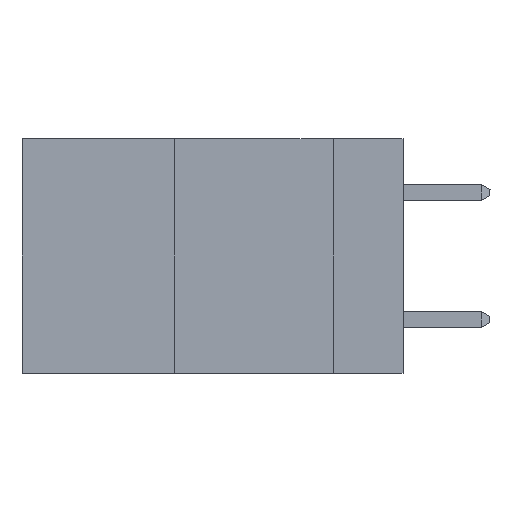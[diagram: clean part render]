
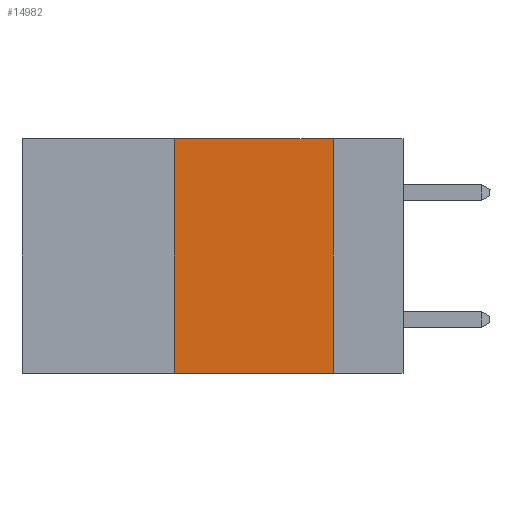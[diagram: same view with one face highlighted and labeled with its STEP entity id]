
A CAD part, left-side view. The second image highlights one B-rep face of the part: STEP entity #14982.
In plain terms, the highlighted planar face has unit normal (-1, 0, 0).
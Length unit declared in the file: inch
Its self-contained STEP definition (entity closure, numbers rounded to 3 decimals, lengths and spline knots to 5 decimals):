
#1082 = AXIS2_PLACEMENT_3D ( 'NONE', #10005, #19451, #3725 ) ;
#1822 = CARTESIAN_POINT ( 'NONE',  ( 0., 0.11, 0. ) ) ;
#2431 = DIRECTION ( 'NONE',  ( 0., -1., 0. ) ) ;
#2682 = EDGE_CURVE ( 'NONE', #5881, #14413, #19854, .T. ) ;
#3580 = CARTESIAN_POINT ( 'NONE',  ( 0., 0.11, -0.37 ) ) ;
#3661 = PLANE ( 'NONE',  #1082 ) ;
#3725 = DIRECTION ( 'NONE',  ( 0., 0., -1. ) ) ;
#3844 = LINE ( 'NONE', #13493, #9092 ) ;
#3905 = FACE_OUTER_BOUND ( 'NONE', #15413, .T. ) ;
#4146 = CARTESIAN_POINT ( 'NONE',  ( 0., 0.6, 0. ) ) ;
#5061 = VECTOR ( 'NONE', #5897, 39.37008 ) ;
#5077 = ORIENTED_EDGE ( 'NONE', *, *, #10117, .F. ) ;
#5511 = DIRECTION ( 'NONE',  ( 0., 0., -1. ) ) ;
#5881 = VERTEX_POINT ( 'NONE', #6553 ) ;
#5897 = DIRECTION ( 'NONE',  ( 0., -1., 0. ) ) ;
#6307 = CARTESIAN_POINT ( 'NONE',  ( 0., 0.36, 0. ) ) ;
#6553 = CARTESIAN_POINT ( 'NONE',  ( 0., 0.36, 0. ) ) ;
#8255 = EDGE_CURVE ( 'NONE', #11700, #13579, #10612, .T. ) ;
#8374 = DIRECTION ( 'NONE',  ( 0., 0., 1. ) ) ;
#9092 = VECTOR ( 'NONE', #5511, 39.37008 ) ;
#10005 = CARTESIAN_POINT ( 'NONE',  ( 0., 0.6, 0. ) ) ;
#10117 = EDGE_CURVE ( 'NONE', #14413, #13579, #3844, .T. ) ;
#10612 = LINE ( 'NONE', #15279, #5061 ) ;
#11083 = ORIENTED_EDGE ( 'NONE', *, *, #2682, .F. ) ;
#11700 = VERTEX_POINT ( 'NONE', #14777 ) ;
#12066 = ORIENTED_EDGE ( 'NONE', *, *, #8255, .T. ) ;
#12709 = VECTOR ( 'NONE', #8374, 39.37008 ) ;
#13493 = CARTESIAN_POINT ( 'NONE',  ( 0., 0.11, 0. ) ) ;
#13579 = VERTEX_POINT ( 'NONE', #3580 ) ;
#14216 = EDGE_CURVE ( 'NONE', #11700, #5881, #16455, .T. ) ;
#14413 = VERTEX_POINT ( 'NONE', #1822 ) ;
#14777 = CARTESIAN_POINT ( 'NONE',  ( 0., 0.36, -0.37 ) ) ;
#14982 = ADVANCED_FACE ( 'NONE', ( #3905 ), #3661, .F. ) ;
#15279 = CARTESIAN_POINT ( 'NONE',  ( 0., 0.6, -0.37 ) ) ;
#15314 = ORIENTED_EDGE ( 'NONE', *, *, #14216, .F. ) ;
#15413 = EDGE_LOOP ( 'NONE', ( #5077, #11083, #15314, #12066 ) ) ;
#16455 = LINE ( 'NONE', #6307, #12709 ) ;
#16868 = VECTOR ( 'NONE', #2431, 39.37008 ) ;
#19451 = DIRECTION ( 'NONE',  ( 1., 0., 0. ) ) ;
#19854 = LINE ( 'NONE', #4146, #16868 ) ;
